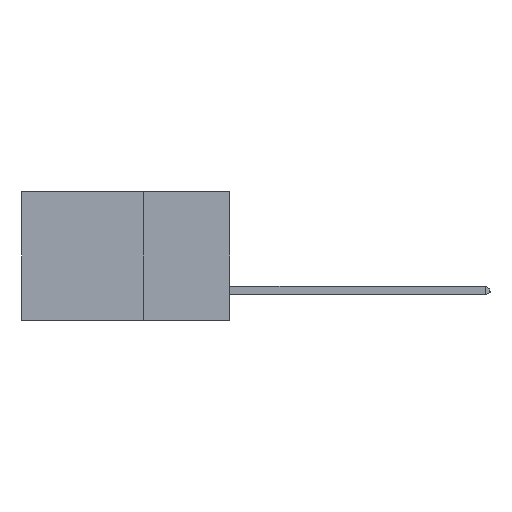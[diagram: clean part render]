
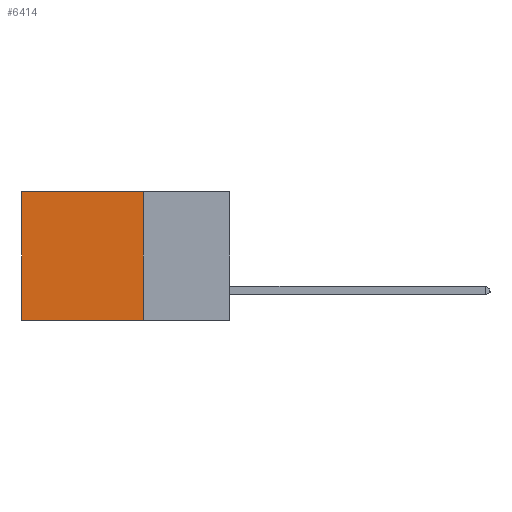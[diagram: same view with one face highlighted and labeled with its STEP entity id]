
A CAD part, left-side view. The second image highlights one B-rep face of the part: STEP entity #6414.
In plain terms, the highlighted planar face has unit normal (-1, 0, 0).
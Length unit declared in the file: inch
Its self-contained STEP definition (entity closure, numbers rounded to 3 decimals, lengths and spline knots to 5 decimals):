
#830 = VECTOR ( 'NONE', #13302, 39.37008 ) ;
#928 = VERTEX_POINT ( 'NONE', #4748 ) ;
#1400 = LINE ( 'NONE', #4165, #10109 ) ;
#1533 = LINE ( 'NONE', #4364, #830 ) ;
#1750 = VERTEX_POINT ( 'NONE', #11719 ) ;
#2267 = CARTESIAN_POINT ( 'NONE',  ( 0.298, 0.6, 0. ) ) ;
#3192 = VERTEX_POINT ( 'NONE', #2267 ) ;
#4165 = CARTESIAN_POINT ( 'NONE',  ( 0.298, 0.25, -0.37 ) ) ;
#4182 = LINE ( 'NONE', #13698, #4880 ) ;
#4364 = CARTESIAN_POINT ( 'NONE',  ( 0.298, 0.6, 0. ) ) ;
#4748 = CARTESIAN_POINT ( 'NONE',  ( 0.298, 0.25, -0.37 ) ) ;
#4880 = VECTOR ( 'NONE', #9272, 39.37008 ) ;
#5107 = AXIS2_PLACEMENT_3D ( 'NONE', #6908, #7942, #8034 ) ;
#5159 = DIRECTION ( 'NONE',  ( 0., 1., 0. ) ) ;
#6414 = ADVANCED_FACE ( 'NONE', ( #11382 ), #7989, .F. ) ;
#6739 = ORIENTED_EDGE ( 'NONE', *, *, #11545, .T. ) ;
#6908 = CARTESIAN_POINT ( 'NONE',  ( 0.298, 0.25, 0. ) ) ;
#6996 = EDGE_CURVE ( 'NONE', #11403, #928, #4182, .T. ) ;
#7246 = EDGE_CURVE ( 'NONE', #928, #1750, #1400, .T. ) ;
#7527 = CARTESIAN_POINT ( 'NONE',  ( 0.298, 0.25, 0. ) ) ;
#7942 = DIRECTION ( 'NONE',  ( 1., 0., 0. ) ) ;
#7989 = PLANE ( 'NONE',  #5107 ) ;
#8034 = DIRECTION ( 'NONE',  ( 0., 0., -1. ) ) ;
#8235 = VECTOR ( 'NONE', #5159, 39.37008 ) ;
#8531 = EDGE_CURVE ( 'NONE', #3192, #1750, #1533, .T. ) ;
#8554 = EDGE_LOOP ( 'NONE', ( #9583, #14316, #13692, #6739 ) ) ;
#9272 = DIRECTION ( 'NONE',  ( 0., 0., -1. ) ) ;
#9583 = ORIENTED_EDGE ( 'NONE', *, *, #8531, .T. ) ;
#10109 = VECTOR ( 'NONE', #14083, 39.37008 ) ;
#10340 = LINE ( 'NONE', #7527, #8235 ) ;
#10487 = CARTESIAN_POINT ( 'NONE',  ( 0.298, 0.25, 0. ) ) ;
#11382 = FACE_OUTER_BOUND ( 'NONE', #8554, .T. ) ;
#11403 = VERTEX_POINT ( 'NONE', #10487 ) ;
#11545 = EDGE_CURVE ( 'NONE', #11403, #3192, #10340, .T. ) ;
#11719 = CARTESIAN_POINT ( 'NONE',  ( 0.298, 0.6, -0.37 ) ) ;
#13302 = DIRECTION ( 'NONE',  ( 0., 0., -1. ) ) ;
#13692 = ORIENTED_EDGE ( 'NONE', *, *, #6996, .F. ) ;
#13698 = CARTESIAN_POINT ( 'NONE',  ( 0.298, 0.25, 0. ) ) ;
#14083 = DIRECTION ( 'NONE',  ( 0., 1., 0. ) ) ;
#14316 = ORIENTED_EDGE ( 'NONE', *, *, #7246, .F. ) ;
